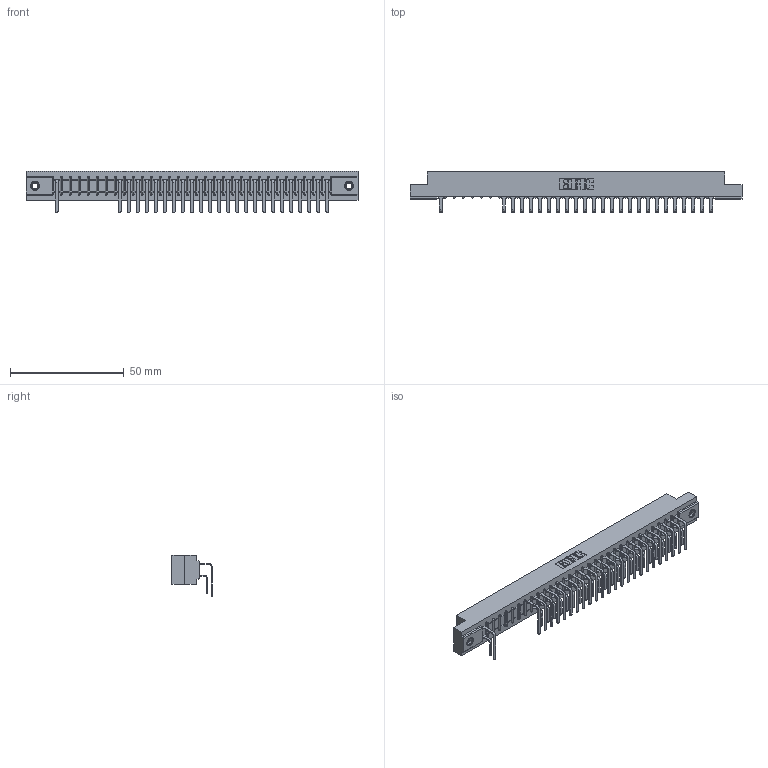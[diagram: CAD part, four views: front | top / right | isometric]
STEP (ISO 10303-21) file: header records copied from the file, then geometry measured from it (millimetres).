
FILE_DESCRIPTION (( 'STEP AP203' ), '1' );
FILE_NAME ('307-031-559-107.STEP', '2018-08-04T20:37:18', ( '' ), ( '' ), 'SwSTEP 2.0', 'SolidWorks 2016', '' );
FILE_SCHEMA (( 'CONFIG_CONTROL_DESIGN' ));
Length unit declared in the file: inch
Products named in the file (5): 307-290-001_558 559 - 1 (Single); 307-290-001_559 - 2 (Single); 345-250-001_345-250-005-103; 307-031-559-107; 307 Part_.156 Dia Mounting Holes
Assembly tree (52 placements, depth 2):
  307-031-559-107
    307 Part_.156 Dia Mounting Holes
    307-290-001_558 559 - 1 (Single)  x24
    307-290-001_559 - 2 (Single)  x25
    345-250-001_345-250-005-103  x2
Bounding box: 145.85 x 17.69 x 18.07 mm (x, y, z)
Volume: 15468.2 mm3; surface area: 18908.5 mm2
Topology: 52 solids, 52 shells, 2790 faces, 7833 edges, 5062 vertices
Faces by surface type: plane 1797, cylinder 913, sphere 64, cone 12, torus 4
Entity records: 31140 total; most frequent: CARTESIAN_POINT 5139, ORIENTED_EDGE 5098, DIRECTION 5033, EDGE_CURVE 2549, LINE 1949, VECTOR 1949, VERTEX_POINT 1648, AXIS2_PLACEMENT_3D 1542
